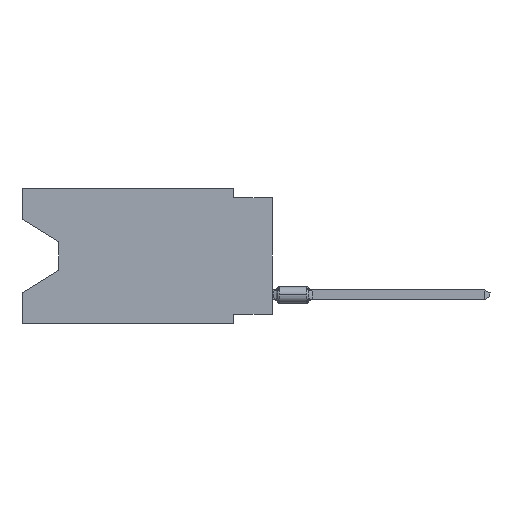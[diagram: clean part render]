
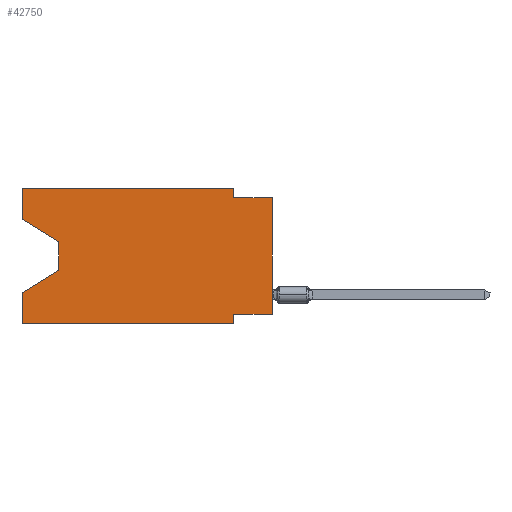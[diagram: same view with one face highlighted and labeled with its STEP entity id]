
A CAD part, left-side view. The second image highlights one B-rep face of the part: STEP entity #42750.
In plain terms, the highlighted planar face has unit normal (-1, 0, 0).
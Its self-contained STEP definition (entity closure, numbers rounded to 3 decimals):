
#110 = EDGE_CURVE ( 'NONE', #48690, #42597, #1237, .T. ) ;
#254 = ORIENTED_EDGE ( 'NONE', *, *, #1778, .F. ) ;
#1237 = LINE ( 'NONE', #48964, #37922 ) ;
#1778 = EDGE_CURVE ( 'NONE', #17518, #52095, #5578, .T. ) ;
#1947 = VERTEX_POINT ( 'NONE', #22006 ) ;
#2077 = EDGE_CURVE ( 'NONE', #28290, #48690, #47562, .T. ) ;
#2269 = ORIENTED_EDGE ( 'NONE', *, *, #25962, .T. ) ;
#2661 = EDGE_CURVE ( 'NONE', #14853, #3882, #7757, .T. ) ;
#2680 = VECTOR ( 'NONE', #51628, 1000. ) ;
#2935 = ORIENTED_EDGE ( 'NONE', *, *, #23099, .F. ) ;
#3379 = VECTOR ( 'NONE', #20017, 1000. ) ;
#3770 = CARTESIAN_POINT ( 'NONE',  ( 0., 0., -8.255 ) ) ;
#3882 = VERTEX_POINT ( 'NONE', #49540 ) ;
#5578 = LINE ( 'NONE', #50394, #8153 ) ;
#5841 = EDGE_CURVE ( 'NONE', #3882, #6512, #15752, .T. ) ;
#6310 = LINE ( 'NONE', #34855, #2680 ) ;
#6512 = VERTEX_POINT ( 'NONE', #10540 ) ;
#7457 = LINE ( 'NONE', #15483, #28647 ) ;
#7757 = LINE ( 'NONE', #3770, #17656 ) ;
#8153 = VECTOR ( 'NONE', #36222, 1000. ) ;
#8808 = VECTOR ( 'NONE', #17087, 1000. ) ;
#8958 = EDGE_LOOP ( 'NONE', ( #31806, #12122, #15334, #50303, #2269, #32817, #24383, #31427, #45575, #2935, #46862, #254 ) ) ;
#9128 = DIRECTION ( 'NONE',  ( 0., -1., 0. ) ) ;
#9309 = LINE ( 'NONE', #13588, #8808 ) ;
#9451 = CARTESIAN_POINT ( 'NONE',  ( 0., 16.383, 0. ) ) ;
#9871 = DIRECTION ( 'NONE',  ( 0., 0., -1. ) ) ;
#10540 = CARTESIAN_POINT ( 'NONE',  ( 0., 2.54, -8.89 ) ) ;
#11496 = VECTOR ( 'NONE', #12125, 1000. ) ;
#12122 = ORIENTED_EDGE ( 'NONE', *, *, #2077, .T. ) ;
#12125 = DIRECTION ( 'NONE',  ( 0., -0.855, -0.519 ) ) ;
#12131 = LINE ( 'NONE', #28391, #22659 ) ;
#13588 = CARTESIAN_POINT ( 'NONE',  ( 0., 2.54, 0. ) ) ;
#14820 = CARTESIAN_POINT ( 'NONE',  ( 0., 16.383, 0. ) ) ;
#14853 = VERTEX_POINT ( 'NONE', #27740 ) ;
#15025 = CARTESIAN_POINT ( 'NONE',  ( 0., 13.97, -3.505 ) ) ;
#15334 = ORIENTED_EDGE ( 'NONE', *, *, #110, .T. ) ;
#15483 = CARTESIAN_POINT ( 'NONE',  ( 0., 0., -0.635 ) ) ;
#15752 = LINE ( 'NONE', #49062, #3379 ) ;
#15803 = CARTESIAN_POINT ( 'NONE',  ( 0., 16.383, -8.89 ) ) ;
#17087 = DIRECTION ( 'NONE',  ( 0., 0., -1. ) ) ;
#17508 = DIRECTION ( 'NONE',  ( 0., 0.855, -0.519 ) ) ;
#17518 = VERTEX_POINT ( 'NONE', #23942 ) ;
#17656 = VECTOR ( 'NONE', #24297, 1000. ) ;
#17964 = CARTESIAN_POINT ( 'NONE',  ( 0., 16.383, 0. ) ) ;
#18248 = EDGE_CURVE ( 'NONE', #22517, #26143, #7457, .T. ) ;
#19097 = LINE ( 'NONE', #14820, #47133 ) ;
#20017 = DIRECTION ( 'NONE',  ( 0., 0., -1. ) ) ;
#20415 = DIRECTION ( 'NONE',  ( 0., -1., 0. ) ) ;
#20543 = VECTOR ( 'NONE', #9128, 1000. ) ;
#22006 = CARTESIAN_POINT ( 'NONE',  ( 0., 2.54, 0. ) ) ;
#22517 = VERTEX_POINT ( 'NONE', #45152 ) ;
#22659 = VECTOR ( 'NONE', #20415, 1000. ) ;
#23099 = EDGE_CURVE ( 'NONE', #1947, #22517, #9309, .T. ) ;
#23120 = EDGE_CURVE ( 'NONE', #25147, #42597, #19097, .T. ) ;
#23942 = CARTESIAN_POINT ( 'NONE',  ( 0., 16.383, -2.038 ) ) ;
#24196 = CARTESIAN_POINT ( 'NONE',  ( 0., 13.97, -3.505 ) ) ;
#24297 = DIRECTION ( 'NONE',  ( 0., 1., 0. ) ) ;
#24383 = ORIENTED_EDGE ( 'NONE', *, *, #2661, .F. ) ;
#24680 = EDGE_CURVE ( 'NONE', #17518, #28290, #45450, .T. ) ;
#25147 = VERTEX_POINT ( 'NONE', #15803 ) ;
#25685 = LINE ( 'NONE', #17964, #20543 ) ;
#25962 = EDGE_CURVE ( 'NONE', #25147, #6512, #12131, .T. ) ;
#26143 = VERTEX_POINT ( 'NONE', #44061 ) ;
#26860 = DIRECTION ( 'NONE',  ( 1., 0., 0. ) ) ;
#27740 = CARTESIAN_POINT ( 'NONE',  ( 0., 0., -8.255 ) ) ;
#28290 = VERTEX_POINT ( 'NONE', #24196 ) ;
#28391 = CARTESIAN_POINT ( 'NONE',  ( 0., 16.383, -8.89 ) ) ;
#28647 = VECTOR ( 'NONE', #52260, 1000. ) ;
#30146 = FACE_OUTER_BOUND ( 'NONE', #8958, .T. ) ;
#31427 = ORIENTED_EDGE ( 'NONE', *, *, #39510, .T. ) ;
#31806 = ORIENTED_EDGE ( 'NONE', *, *, #24680, .T. ) ;
#32817 = ORIENTED_EDGE ( 'NONE', *, *, #5841, .F. ) ;
#33185 = CARTESIAN_POINT ( 'NONE',  ( 0., 13.97, -5.385 ) ) ;
#34855 = CARTESIAN_POINT ( 'NONE',  ( 0., 0., 0. ) ) ;
#36222 = DIRECTION ( 'NONE',  ( 0., 0., 1. ) ) ;
#36681 = CARTESIAN_POINT ( 'NONE',  ( 0., 16.383, -2.038 ) ) ;
#37922 = VECTOR ( 'NONE', #17508, 1000. ) ;
#39034 = EDGE_CURVE ( 'NONE', #52095, #1947, #25685, .T. ) ;
#39321 = DIRECTION ( 'NONE',  ( 0., 0., -1. ) ) ;
#39510 = EDGE_CURVE ( 'NONE', #14853, #26143, #6310, .T. ) ;
#39618 = DIRECTION ( 'NONE',  ( 0., 0., 1. ) ) ;
#42597 = VERTEX_POINT ( 'NONE', #48341 ) ;
#42750 = ADVANCED_FACE ( 'NONE', ( #30146 ), #50442, .F. ) ;
#44061 = CARTESIAN_POINT ( 'NONE',  ( 0., 0., -0.635 ) ) ;
#45152 = CARTESIAN_POINT ( 'NONE',  ( 0., 2.54, -0.635 ) ) ;
#45450 = LINE ( 'NONE', #36681, #11496 ) ;
#45575 = ORIENTED_EDGE ( 'NONE', *, *, #18248, .F. ) ;
#46862 = ORIENTED_EDGE ( 'NONE', *, *, #39034, .F. ) ;
#47133 = VECTOR ( 'NONE', #39618, 1000. ) ;
#47351 = VECTOR ( 'NONE', #39321, 1000. ) ;
#47562 = LINE ( 'NONE', #15025, #47351 ) ;
#48341 = CARTESIAN_POINT ( 'NONE',  ( 0., 16.383, -6.852 ) ) ;
#48690 = VERTEX_POINT ( 'NONE', #33185 ) ;
#48964 = CARTESIAN_POINT ( 'NONE',  ( 0., 13.97, -5.385 ) ) ;
#49062 = CARTESIAN_POINT ( 'NONE',  ( 0., 2.54, -8.89 ) ) ;
#49540 = CARTESIAN_POINT ( 'NONE',  ( 0., 2.54, -8.255 ) ) ;
#50303 = ORIENTED_EDGE ( 'NONE', *, *, #23120, .F. ) ;
#50394 = CARTESIAN_POINT ( 'NONE',  ( 0., 16.383, 0. ) ) ;
#50442 = PLANE ( 'NONE',  #50638 ) ;
#50638 = AXIS2_PLACEMENT_3D ( 'NONE', #51397, #26860, #9871 ) ;
#51397 = CARTESIAN_POINT ( 'NONE',  ( 0., 16.383, 0. ) ) ;
#51628 = DIRECTION ( 'NONE',  ( 0., 0., 1. ) ) ;
#52095 = VERTEX_POINT ( 'NONE', #9451 ) ;
#52260 = DIRECTION ( 'NONE',  ( 0., -1., 0. ) ) ;
